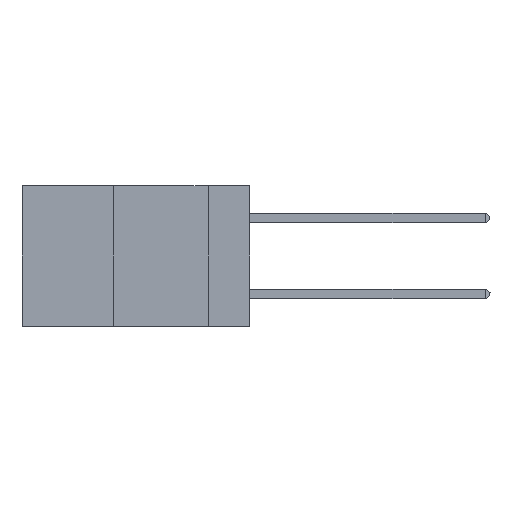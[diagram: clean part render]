
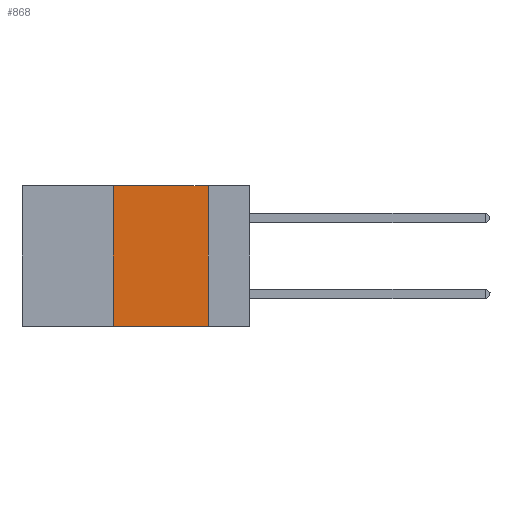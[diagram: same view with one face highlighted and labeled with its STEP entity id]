
A CAD part, left-side view. The second image highlights one B-rep face of the part: STEP entity #868.
In plain terms, the highlighted planar face has unit normal (-1, 0, 0).
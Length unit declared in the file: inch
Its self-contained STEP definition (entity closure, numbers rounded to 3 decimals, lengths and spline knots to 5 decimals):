
#156 = EDGE_CURVE ( 'NONE', #586, #13753, #20288, .T. ) ;
#586 = VERTEX_POINT ( 'NONE', #19278 ) ;
#868 = ADVANCED_FACE ( 'NONE', ( #21680 ), #21692, .F. ) ;
#1274 = DIRECTION ( 'NONE',  ( 1., 0., 0. ) ) ;
#2843 = EDGE_CURVE ( 'NONE', #13753, #21975, #4016, .T. ) ;
#3151 = CARTESIAN_POINT ( 'NONE',  ( 0., 0.36, 0. ) ) ;
#3777 = VECTOR ( 'NONE', #16047, 39.37008 ) ;
#4016 = LINE ( 'NONE', #13343, #13874 ) ;
#5580 = DIRECTION ( 'NONE',  ( 0., -1., 0. ) ) ;
#5848 = AXIS2_PLACEMENT_3D ( 'NONE', #10359, #1274, #23314 ) ;
#6795 = EDGE_LOOP ( 'NONE', ( #11022, #19126, #14857, #18280 ) ) ;
#7308 = VERTEX_POINT ( 'NONE', #9671 ) ;
#9671 = CARTESIAN_POINT ( 'NONE',  ( 0., 0.11, -0.37 ) ) ;
#9718 = VECTOR ( 'NONE', #17691, 39.37008 ) ;
#10359 = CARTESIAN_POINT ( 'NONE',  ( 0., 0.6, 0. ) ) ;
#11022 = ORIENTED_EDGE ( 'NONE', *, *, #21291, .F. ) ;
#11583 = CARTESIAN_POINT ( 'NONE',  ( 0., 0.11, 0. ) ) ;
#12053 = LINE ( 'NONE', #16171, #9718 ) ;
#13113 = CARTESIAN_POINT ( 'NONE',  ( 0., 0.6, -0.37 ) ) ;
#13343 = CARTESIAN_POINT ( 'NONE',  ( 0., 0.6, 0. ) ) ;
#13646 = DIRECTION ( 'NONE',  ( 0., -1., 0. ) ) ;
#13753 = VERTEX_POINT ( 'NONE', #18358 ) ;
#13874 = VECTOR ( 'NONE', #13646, 39.37008 ) ;
#14857 = ORIENTED_EDGE ( 'NONE', *, *, #156, .F. ) ;
#16047 = DIRECTION ( 'NONE',  ( 0., 0., 1. ) ) ;
#16171 = CARTESIAN_POINT ( 'NONE',  ( 0., 0.11, 0. ) ) ;
#17691 = DIRECTION ( 'NONE',  ( 0., 0., -1. ) ) ;
#17784 = LINE ( 'NONE', #13113, #19535 ) ;
#18280 = ORIENTED_EDGE ( 'NONE', *, *, #23669, .T. ) ;
#18358 = CARTESIAN_POINT ( 'NONE',  ( 0., 0.36, 0. ) ) ;
#19126 = ORIENTED_EDGE ( 'NONE', *, *, #2843, .F. ) ;
#19278 = CARTESIAN_POINT ( 'NONE',  ( 0., 0.36, -0.37 ) ) ;
#19535 = VECTOR ( 'NONE', #5580, 39.37008 ) ;
#20288 = LINE ( 'NONE', #3151, #3777 ) ;
#21291 = EDGE_CURVE ( 'NONE', #21975, #7308, #12053, .T. ) ;
#21680 = FACE_OUTER_BOUND ( 'NONE', #6795, .T. ) ;
#21692 = PLANE ( 'NONE',  #5848 ) ;
#21975 = VERTEX_POINT ( 'NONE', #11583 ) ;
#23314 = DIRECTION ( 'NONE',  ( 0., 0., -1. ) ) ;
#23669 = EDGE_CURVE ( 'NONE', #586, #7308, #17784, .T. ) ;
